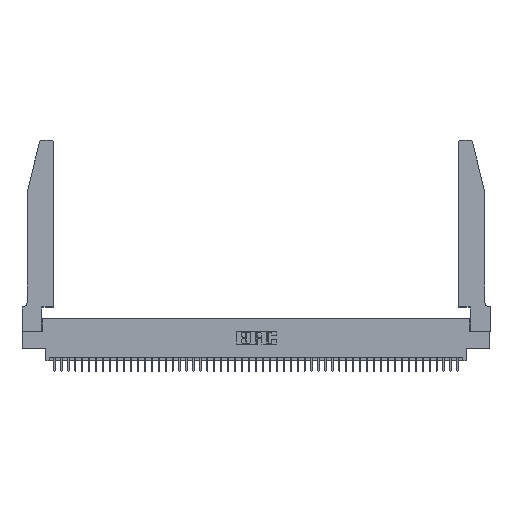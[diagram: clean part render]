
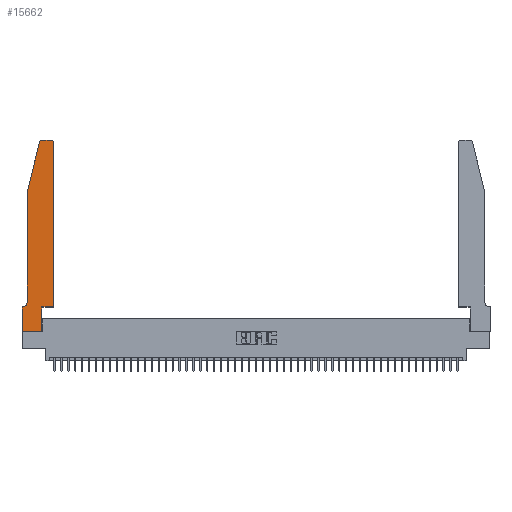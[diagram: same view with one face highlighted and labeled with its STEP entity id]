
A CAD part, top view. The second image highlights one B-rep face of the part: STEP entity #15662.
In plain terms, the highlighted planar face has unit normal (0, 0, 1).
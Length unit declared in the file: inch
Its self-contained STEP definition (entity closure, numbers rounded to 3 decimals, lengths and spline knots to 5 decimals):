
#830 = LINE ( 'NONE', #31340, #36921 ) ;
#2103 = LINE ( 'NONE', #19491, #45922 ) ;
#2302 = VECTOR ( 'NONE', #43194, 39.37008 ) ;
#2687 = FACE_OUTER_BOUND ( 'NONE', #5751, .T. ) ;
#3372 = ORIENTED_EDGE ( 'NONE', *, *, #4208, .T. ) ;
#4156 = VECTOR ( 'NONE', #9865, 39.37008 ) ;
#4208 = EDGE_CURVE ( 'NONE', #34705, #28735, #33893, .T. ) ;
#4461 = VERTEX_POINT ( 'NONE', #4802 ) ;
#4517 = CARTESIAN_POINT ( 'NONE',  ( 0., 0., 0.37 ) ) ;
#4721 = LINE ( 'NONE', #32686, #16015 ) ;
#4802 = CARTESIAN_POINT ( 'NONE',  ( 0.2865, 0.35, 0.37 ) ) ;
#4883 = VERTEX_POINT ( 'NONE', #27099 ) ;
#5751 = EDGE_LOOP ( 'NONE', ( #11822, #3372, #23961, #20965, #10803, #37024, #38741, #24887, #23254, #46783, #36193, #20915 ) ) ;
#5983 = CARTESIAN_POINT ( 'NONE',  ( 0.2865, 0., 0.37 ) ) ;
#5999 = VERTEX_POINT ( 'NONE', #39484 ) ;
#7928 = EDGE_CURVE ( 'NONE', #19121, #35717, #14262, .T. ) ;
#8121 = CARTESIAN_POINT ( 'NONE',  ( 0.0055, 0.42, 0.37 ) ) ;
#8532 = EDGE_CURVE ( 'NONE', #23166, #33322, #35459, .T. ) ;
#8563 = DIRECTION ( 'NONE',  ( 1., 0., 0. ) ) ;
#9084 = CARTESIAN_POINT ( 'NONE',  ( 0., 0.35, 0.37 ) ) ;
#9547 = CIRCLE ( 'NONE', #25857, 0.07 ) ;
#9865 = DIRECTION ( 'NONE',  ( 0., 1., 0. ) ) ;
#10506 = CARTESIAN_POINT ( 'NONE',  ( 0.25487, 2.72718, 0.37 ) ) ;
#10803 = ORIENTED_EDGE ( 'NONE', *, *, #31852, .T. ) ;
#11392 = VECTOR ( 'NONE', #8563, 39.37008 ) ;
#11822 = ORIENTED_EDGE ( 'NONE', *, *, #24183, .T. ) ;
#14262 = LINE ( 'NONE', #24568, #4156 ) ;
#14537 = CARTESIAN_POINT ( 'NONE',  ( 0.4505, 0.35, 0.37 ) ) ;
#15662 = ADVANCED_FACE ( 'NONE', ( #2687 ), #24101, .T. ) ;
#15822 = LINE ( 'NONE', #23392, #33586 ) ;
#16015 = VECTOR ( 'NONE', #25388, 39.37008 ) ;
#16402 = EDGE_CURVE ( 'NONE', #28735, #23166, #830, .T. ) ;
#19121 = VERTEX_POINT ( 'NONE', #14537 ) ;
#19491 = CARTESIAN_POINT ( 'NONE',  ( 0.2865, 0.35, 0.37 ) ) ;
#20365 = DIRECTION ( 'NONE',  ( 1., 0., 0. ) ) ;
#20915 = ORIENTED_EDGE ( 'NONE', *, *, #25154, .T. ) ;
#20965 = ORIENTED_EDGE ( 'NONE', *, *, #8532, .T. ) ;
#21935 = EDGE_CURVE ( 'NONE', #45559, #4461, #2103, .T. ) ;
#22253 = VECTOR ( 'NONE', #42059, 39.37008 ) ;
#22630 = VECTOR ( 'NONE', #39330, 39.37008 ) ;
#23166 = VERTEX_POINT ( 'NONE', #34927 ) ;
#23254 = ORIENTED_EDGE ( 'NONE', *, *, #21935, .T. ) ;
#23392 = CARTESIAN_POINT ( 'NONE',  ( 0.0755, 0.35, 0.37 ) ) ;
#23673 = CARTESIAN_POINT ( 'NONE',  ( 0.0755, 2., 0.37 ) ) ;
#23705 = DIRECTION ( 'NONE',  ( -0.239, -0.971, 0. ) ) ;
#23961 = ORIENTED_EDGE ( 'NONE', *, *, #16402, .T. ) ;
#24019 = EDGE_CURVE ( 'NONE', #4461, #19121, #27938, .T. ) ;
#24101 = PLANE ( 'NONE',  #27848 ) ;
#24183 = EDGE_CURVE ( 'NONE', #5999, #34705, #32710, .T. ) ;
#24408 = CARTESIAN_POINT ( 'NONE',  ( 0.284, 2.75, 0.37 ) ) ;
#24568 = CARTESIAN_POINT ( 'NONE',  ( 0.4505, 0.35, 0.37 ) ) ;
#24887 = ORIENTED_EDGE ( 'NONE', *, *, #42997, .T. ) ;
#25154 = EDGE_CURVE ( 'NONE', #35717, #5999, #40847, .T. ) ;
#25388 = DIRECTION ( 'NONE',  ( 1., 0., 0. ) ) ;
#25857 = AXIS2_PLACEMENT_3D ( 'NONE', #8121, #30598, #45821 ) ;
#25858 = CARTESIAN_POINT ( 'NONE',  ( 0.4505, 2.72, 0.37 ) ) ;
#26515 = CARTESIAN_POINT ( 'NONE',  ( 0., 0.35, 0.37 ) ) ;
#27099 = CARTESIAN_POINT ( 'NONE',  ( 0., 0., 0.37 ) ) ;
#27171 = CARTESIAN_POINT ( 'NONE',  ( 0.0755, 0.42, 0.37 ) ) ;
#27848 = AXIS2_PLACEMENT_3D ( 'NONE', #9084, #32243, #46948 ) ;
#27935 = DIRECTION ( 'NONE',  ( 0., 0., 1. ) ) ;
#27938 = LINE ( 'NONE', #31362, #11392 ) ;
#28735 = VERTEX_POINT ( 'NONE', #10506 ) ;
#28930 = EDGE_CURVE ( 'NONE', #41904, #4883, #38251, .T. ) ;
#29466 = AXIS2_PLACEMENT_3D ( 'NONE', #39203, #27935, #20365 ) ;
#30598 = DIRECTION ( 'NONE',  ( 0., 0., -1. ) ) ;
#30849 = DIRECTION ( 'NONE',  ( -1., 0., 0. ) ) ;
#31340 = CARTESIAN_POINT ( 'NONE',  ( 0.0755, 2., 0.37 ) ) ;
#31362 = CARTESIAN_POINT ( 'NONE',  ( 0.4505, 0.35, 0.37 ) ) ;
#31852 = EDGE_CURVE ( 'NONE', #33322, #42859, #9547, .T. ) ;
#32243 = DIRECTION ( 'NONE',  ( 0., 0., 1. ) ) ;
#32686 = CARTESIAN_POINT ( 'NONE',  ( 0., 0., 0.37 ) ) ;
#32710 = LINE ( 'NONE', #46761, #22630 ) ;
#33322 = VERTEX_POINT ( 'NONE', #27171 ) ;
#33586 = VECTOR ( 'NONE', #30849, 39.37008 ) ;
#33893 = CIRCLE ( 'NONE', #43970, 0.03 ) ;
#34220 = DIRECTION ( 'NONE',  ( 0., 1., 0. ) ) ;
#34705 = VERTEX_POINT ( 'NONE', #24408 ) ;
#34927 = CARTESIAN_POINT ( 'NONE',  ( 0.0755, 2., 0.37 ) ) ;
#34940 = DIRECTION ( 'NONE',  ( 1., 0., 0. ) ) ;
#35459 = LINE ( 'NONE', #23673, #2302 ) ;
#35717 = VERTEX_POINT ( 'NONE', #25858 ) ;
#36193 = ORIENTED_EDGE ( 'NONE', *, *, #7928, .T. ) ;
#36921 = VECTOR ( 'NONE', #23705, 39.37008 ) ;
#37024 = ORIENTED_EDGE ( 'NONE', *, *, #44715, .T. ) ;
#38100 = CARTESIAN_POINT ( 'NONE',  ( 0.284, 2.72, 0.37 ) ) ;
#38251 = LINE ( 'NONE', #4517, #22253 ) ;
#38588 = DIRECTION ( 'NONE',  ( 0., 0., 1. ) ) ;
#38741 = ORIENTED_EDGE ( 'NONE', *, *, #28930, .T. ) ;
#39203 = CARTESIAN_POINT ( 'NONE',  ( 0.4205, 2.72, 0.37 ) ) ;
#39330 = DIRECTION ( 'NONE',  ( -1., 0., 0. ) ) ;
#39482 = CARTESIAN_POINT ( 'NONE',  ( 0.0055, 0.35, 0.37 ) ) ;
#39484 = CARTESIAN_POINT ( 'NONE',  ( 0.4205, 2.75, 0.37 ) ) ;
#40847 = CIRCLE ( 'NONE', #29466, 0.03 ) ;
#41904 = VERTEX_POINT ( 'NONE', #26515 ) ;
#42059 = DIRECTION ( 'NONE',  ( 0., -1., 0. ) ) ;
#42859 = VERTEX_POINT ( 'NONE', #39482 ) ;
#42997 = EDGE_CURVE ( 'NONE', #4883, #45559, #4721, .T. ) ;
#43194 = DIRECTION ( 'NONE',  ( 0., -1., 0. ) ) ;
#43970 = AXIS2_PLACEMENT_3D ( 'NONE', #38100, #38588, #34940 ) ;
#44715 = EDGE_CURVE ( 'NONE', #42859, #41904, #15822, .T. ) ;
#45559 = VERTEX_POINT ( 'NONE', #5983 ) ;
#45821 = DIRECTION ( 'NONE',  ( -1., 0., 0. ) ) ;
#45922 = VECTOR ( 'NONE', #34220, 39.37008 ) ;
#46761 = CARTESIAN_POINT ( 'NONE',  ( 0.2605, 2.75, 0.37 ) ) ;
#46783 = ORIENTED_EDGE ( 'NONE', *, *, #24019, .T. ) ;
#46948 = DIRECTION ( 'NONE',  ( 1., 0., 0. ) ) ;
